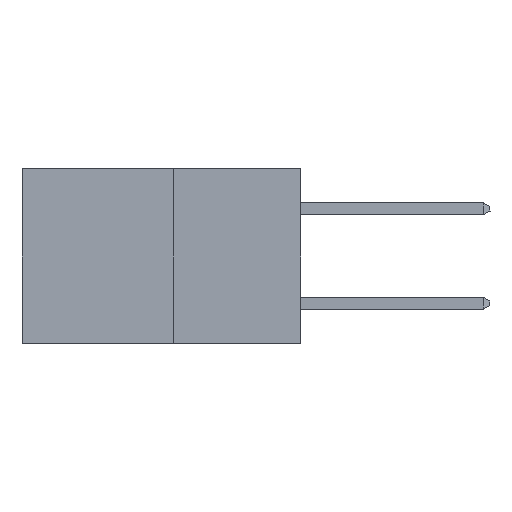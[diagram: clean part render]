
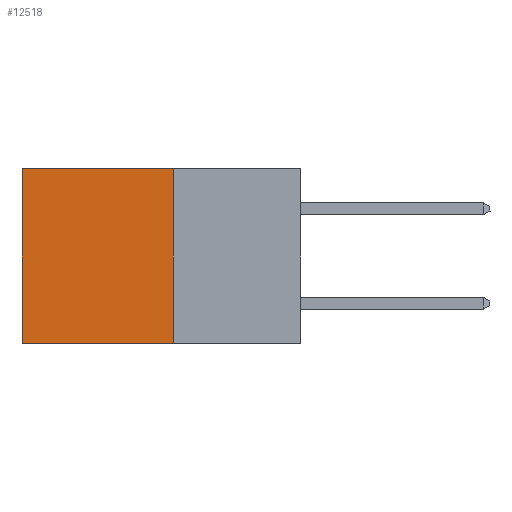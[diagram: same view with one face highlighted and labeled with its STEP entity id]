
A CAD part, left-side view. The second image highlights one B-rep face of the part: STEP entity #12518.
In plain terms, the highlighted planar face has unit normal (-1, 0, 0).
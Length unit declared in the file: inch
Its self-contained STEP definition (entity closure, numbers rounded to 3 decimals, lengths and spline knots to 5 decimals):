
#535 = PLANE ( 'NONE',  #6321 ) ;
#1381 = ORIENTED_EDGE ( 'NONE', *, *, #4658, .F. ) ;
#1480 = VERTEX_POINT ( 'NONE', #5032 ) ;
#1723 = CARTESIAN_POINT ( 'NONE',  ( 0.277, 0.27, 0. ) ) ;
#1814 = LINE ( 'NONE', #5974, #20027 ) ;
#2276 = VECTOR ( 'NONE', #7617, 39.37008 ) ;
#2543 = ORIENTED_EDGE ( 'NONE', *, *, #8897, .F. ) ;
#4107 = VERTEX_POINT ( 'NONE', #12722 ) ;
#4127 = DIRECTION ( 'NONE',  ( 0., 1., 0. ) ) ;
#4194 = DIRECTION ( 'NONE',  ( 1., 0., 0. ) ) ;
#4658 = EDGE_CURVE ( 'NONE', #1480, #4107, #11989, .T. ) ;
#5032 = CARTESIAN_POINT ( 'NONE',  ( 0.277, 0.27, 0. ) ) ;
#5727 = LINE ( 'NONE', #1723, #10605 ) ;
#5819 = CARTESIAN_POINT ( 'NONE',  ( 0.277, 0.59, -0.37 ) ) ;
#5935 = VERTEX_POINT ( 'NONE', #7504 ) ;
#5974 = CARTESIAN_POINT ( 'NONE',  ( 0.277, 0.27, -0.37 ) ) ;
#6121 = VERTEX_POINT ( 'NONE', #11603 ) ;
#6321 = AXIS2_PLACEMENT_3D ( 'NONE', #20495, #4194, #16942 ) ;
#7504 = CARTESIAN_POINT ( 'NONE',  ( 0.277, 0.59, -0.37 ) ) ;
#7617 = DIRECTION ( 'NONE',  ( 0., 0., -1. ) ) ;
#8897 = EDGE_CURVE ( 'NONE', #4107, #5935, #1814, .T. ) ;
#9026 = DIRECTION ( 'NONE',  ( 0., 1., 0. ) ) ;
#9244 = EDGE_CURVE ( 'NONE', #1480, #6121, #5727, .T. ) ;
#10605 = VECTOR ( 'NONE', #9026, 39.37008 ) ;
#11200 = ORIENTED_EDGE ( 'NONE', *, *, #9244, .T. ) ;
#11603 = CARTESIAN_POINT ( 'NONE',  ( 0.277, 0.59, 0. ) ) ;
#11957 = VECTOR ( 'NONE', #22134, 39.37008 ) ;
#11989 = LINE ( 'NONE', #21974, #2276 ) ;
#12518 = ADVANCED_FACE ( 'NONE', ( #12757 ), #535, .F. ) ;
#12722 = CARTESIAN_POINT ( 'NONE',  ( 0.277, 0.27, -0.37 ) ) ;
#12757 = FACE_OUTER_BOUND ( 'NONE', #12793, .T. ) ;
#12793 = EDGE_LOOP ( 'NONE', ( #18495, #2543, #1381, #11200 ) ) ;
#16942 = DIRECTION ( 'NONE',  ( 0., 0., -1. ) ) ;
#18265 = EDGE_CURVE ( 'NONE', #6121, #5935, #22107, .T. ) ;
#18495 = ORIENTED_EDGE ( 'NONE', *, *, #18265, .T. ) ;
#20027 = VECTOR ( 'NONE', #4127, 39.37008 ) ;
#20495 = CARTESIAN_POINT ( 'NONE',  ( 0.277, 0.27, -0.37 ) ) ;
#21974 = CARTESIAN_POINT ( 'NONE',  ( 0.277, 0.27, -0.37 ) ) ;
#22107 = LINE ( 'NONE', #5819, #11957 ) ;
#22134 = DIRECTION ( 'NONE',  ( 0., 0., -1. ) ) ;
